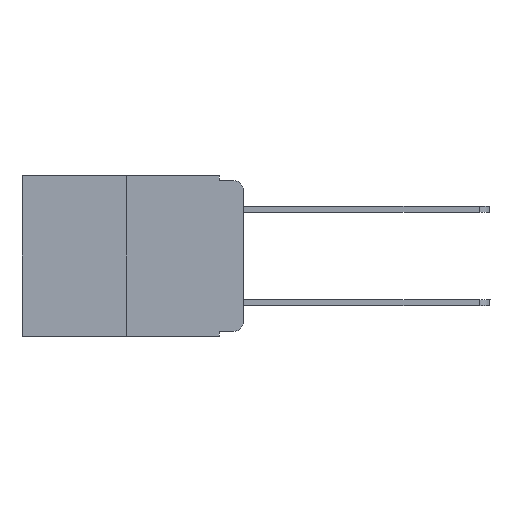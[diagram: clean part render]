
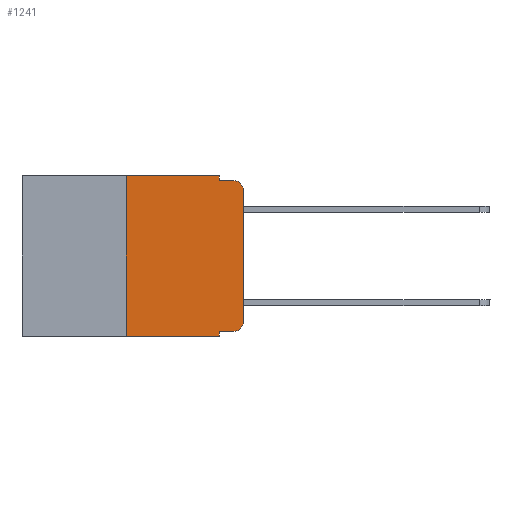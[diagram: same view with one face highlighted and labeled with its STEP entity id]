
A CAD part, left-side view. The second image highlights one B-rep face of the part: STEP entity #1241.
In plain terms, the highlighted planar face has unit normal (-1, 0, 0).
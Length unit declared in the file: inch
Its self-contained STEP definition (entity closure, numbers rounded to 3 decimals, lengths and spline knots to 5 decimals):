
#272 = DIRECTION ( 'NONE',  ( 0., 0., -1. ) ) ;
#542 = CARTESIAN_POINT ( 'NONE',  ( 0., 0., 0. ) ) ;
#988 = VECTOR ( 'NONE', #1507, 39.37008 ) ;
#1004 = DIRECTION ( 'NONE',  ( 0., 0., -1. ) ) ;
#1241 = ADVANCED_FACE ( 'NONE', ( #6812 ), #8051, .F. ) ;
#1386 = EDGE_CURVE ( 'NONE', #6070, #9464, #7295, .T. ) ;
#1507 = DIRECTION ( 'NONE',  ( 0., -1., 0. ) ) ;
#1555 = DIRECTION ( 'NONE',  ( 1., 0., 0. ) ) ;
#1886 = DIRECTION ( 'NONE',  ( 0., 0., -1. ) ) ;
#2210 = VERTEX_POINT ( 'NONE', #7009 ) ;
#2250 = AXIS2_PLACEMENT_3D ( 'NONE', #10566, #4337, #3361 ) ;
#2403 = VERTEX_POINT ( 'NONE', #7424 ) ;
#2834 = VECTOR ( 'NONE', #3728, 39.37008 ) ;
#2870 = CARTESIAN_POINT ( 'NONE',  ( 0., 0.051, 0. ) ) ;
#3030 = CIRCLE ( 'NONE', #2250, 0.02 ) ;
#3047 = CARTESIAN_POINT ( 'NONE',  ( 0., 0.473, 0. ) ) ;
#3065 = VECTOR ( 'NONE', #14542, 39.37008 ) ;
#3181 = DIRECTION ( 'NONE',  ( 0., 0., 1. ) ) ;
#3361 = DIRECTION ( 'NONE',  ( 0., 0., -1. ) ) ;
#3416 = VERTEX_POINT ( 'NONE', #14200 ) ;
#3418 = EDGE_CURVE ( 'NONE', #2403, #14597, #15673, .T. ) ;
#3718 = CARTESIAN_POINT ( 'NONE',  ( 0., 0.051, -0.343 ) ) ;
#3728 = DIRECTION ( 'NONE',  ( 0., -1., 0. ) ) ;
#3736 = VERTEX_POINT ( 'NONE', #5270 ) ;
#4177 = VERTEX_POINT ( 'NONE', #2870 ) ;
#4337 = DIRECTION ( 'NONE',  ( -1., 0., 0. ) ) ;
#4466 = EDGE_LOOP ( 'NONE', ( #6609, #9277, #7119, #6906, #12202, #15919, #4981, #13113, #10848, #13724 ) ) ;
#4705 = CARTESIAN_POINT ( 'NONE',  ( 0., 0.051, -0.01 ) ) ;
#4768 = EDGE_CURVE ( 'NONE', #6070, #7349, #5313, .T. ) ;
#4851 = EDGE_CURVE ( 'NONE', #2210, #2403, #11992, .T. ) ;
#4981 = ORIENTED_EDGE ( 'NONE', *, *, #1386, .T. ) ;
#5131 = CARTESIAN_POINT ( 'NONE',  ( 0., 0.051, -0.333 ) ) ;
#5270 = CARTESIAN_POINT ( 'NONE',  ( 0., 0.051, -0.333 ) ) ;
#5313 = LINE ( 'NONE', #15461, #3065 ) ;
#6070 = VERTEX_POINT ( 'NONE', #9206 ) ;
#6571 = DIRECTION ( 'NONE',  ( 0., 0., -1. ) ) ;
#6609 = ORIENTED_EDGE ( 'NONE', *, *, #4851, .T. ) ;
#6681 = LINE ( 'NONE', #3047, #988 ) ;
#6761 = VECTOR ( 'NONE', #12161, 39.37008 ) ;
#6812 = FACE_OUTER_BOUND ( 'NONE', #4466, .T. ) ;
#6825 = LINE ( 'NONE', #9410, #10203 ) ;
#6906 = ORIENTED_EDGE ( 'NONE', *, *, #11186, .F. ) ;
#7009 = CARTESIAN_POINT ( 'NONE',  ( 0., 0., -0.313 ) ) ;
#7119 = ORIENTED_EDGE ( 'NONE', *, *, #14569, .F. ) ;
#7135 = LINE ( 'NONE', #4705, #6761 ) ;
#7295 = LINE ( 'NONE', #15957, #15191 ) ;
#7349 = VERTEX_POINT ( 'NONE', #15437 ) ;
#7424 = CARTESIAN_POINT ( 'NONE',  ( 0., 0., -0.03 ) ) ;
#7610 = LINE ( 'NONE', #9828, #11982 ) ;
#8051 = PLANE ( 'NONE',  #13584 ) ;
#9204 = CARTESIAN_POINT ( 'NONE',  ( 0., 0.02, -0.03 ) ) ;
#9206 = CARTESIAN_POINT ( 'NONE',  ( 0., 0.25, -0.343 ) ) ;
#9277 = ORIENTED_EDGE ( 'NONE', *, *, #3418, .T. ) ;
#9410 = CARTESIAN_POINT ( 'NONE',  ( 0., 0.051, 0. ) ) ;
#9464 = VERTEX_POINT ( 'NONE', #3718 ) ;
#9481 = DIRECTION ( 'NONE',  ( 0., -1., 0. ) ) ;
#9828 = CARTESIAN_POINT ( 'NONE',  ( 0., 0.051, 0. ) ) ;
#10203 = VECTOR ( 'NONE', #1886, 39.37008 ) ;
#10457 = CARTESIAN_POINT ( 'NONE',  ( 0., 0.473, 0. ) ) ;
#10566 = CARTESIAN_POINT ( 'NONE',  ( 0., 0.02, -0.313 ) ) ;
#10848 = ORIENTED_EDGE ( 'NONE', *, *, #13432, .T. ) ;
#11186 = EDGE_CURVE ( 'NONE', #4177, #3416, #7610, .T. ) ;
#11460 = EDGE_CURVE ( 'NONE', #15864, #2210, #3030, .T. ) ;
#11728 = DIRECTION ( 'NONE',  ( -1., 0., 0. ) ) ;
#11982 = VECTOR ( 'NONE', #1004, 39.37008 ) ;
#11992 = LINE ( 'NONE', #542, #13159 ) ;
#12161 = DIRECTION ( 'NONE',  ( 0., -1., 0. ) ) ;
#12202 = ORIENTED_EDGE ( 'NONE', *, *, #15250, .F. ) ;
#12561 = LINE ( 'NONE', #5131, #2834 ) ;
#13113 = ORIENTED_EDGE ( 'NONE', *, *, #13987, .F. ) ;
#13159 = VECTOR ( 'NONE', #3181, 39.37008 ) ;
#13432 = EDGE_CURVE ( 'NONE', #3736, #15864, #12561, .T. ) ;
#13463 = CARTESIAN_POINT ( 'NONE',  ( 0., 0.02, -0.333 ) ) ;
#13584 = AXIS2_PLACEMENT_3D ( 'NONE', #10457, #1555, #6571 ) ;
#13724 = ORIENTED_EDGE ( 'NONE', *, *, #11460, .T. ) ;
#13968 = CARTESIAN_POINT ( 'NONE',  ( 0., 0.02, -0.01 ) ) ;
#13987 = EDGE_CURVE ( 'NONE', #3736, #9464, #6825, .T. ) ;
#14200 = CARTESIAN_POINT ( 'NONE',  ( 0., 0.051, -0.01 ) ) ;
#14542 = DIRECTION ( 'NONE',  ( 0., 0., 1. ) ) ;
#14569 = EDGE_CURVE ( 'NONE', #3416, #14597, #7135, .T. ) ;
#14597 = VERTEX_POINT ( 'NONE', #13968 ) ;
#15147 = AXIS2_PLACEMENT_3D ( 'NONE', #9204, #11728, #272 ) ;
#15191 = VECTOR ( 'NONE', #9481, 39.37008 ) ;
#15250 = EDGE_CURVE ( 'NONE', #7349, #4177, #6681, .T. ) ;
#15437 = CARTESIAN_POINT ( 'NONE',  ( 0., 0.25, 0. ) ) ;
#15461 = CARTESIAN_POINT ( 'NONE',  ( 0., 0.25, 0. ) ) ;
#15673 = CIRCLE ( 'NONE', #15147, 0.02 ) ;
#15864 = VERTEX_POINT ( 'NONE', #13463 ) ;
#15919 = ORIENTED_EDGE ( 'NONE', *, *, #4768, .F. ) ;
#15957 = CARTESIAN_POINT ( 'NONE',  ( 0., 0.473, -0.343 ) ) ;
